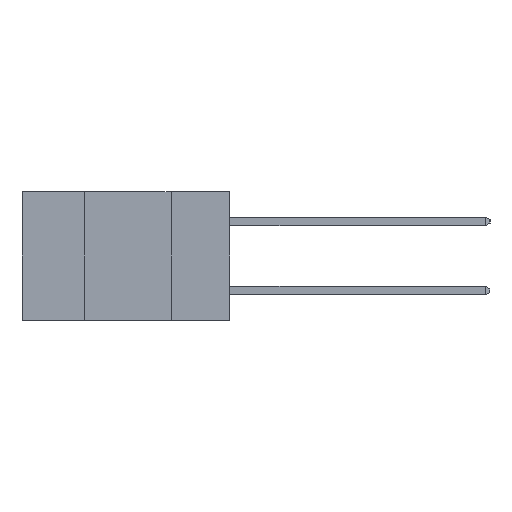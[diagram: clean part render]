
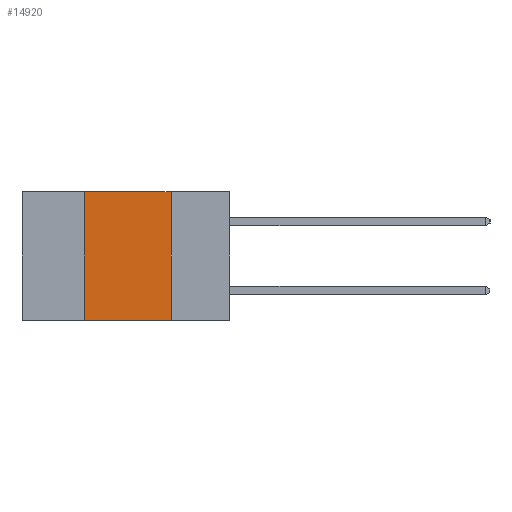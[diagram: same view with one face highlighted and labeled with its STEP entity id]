
A CAD part, left-side view. The second image highlights one B-rep face of the part: STEP entity #14920.
In plain terms, the highlighted planar face has unit normal (-1, 0, 0).
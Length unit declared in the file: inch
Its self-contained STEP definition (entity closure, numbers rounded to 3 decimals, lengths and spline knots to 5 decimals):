
#61 = DIRECTION ( 'NONE',  ( 0., 0., -1. ) ) ;
#88 = CARTESIAN_POINT ( 'NONE',  ( 0., 0.42, 0. ) ) ;
#108 = VERTEX_POINT ( 'NONE', #1842 ) ;
#618 = ORIENTED_EDGE ( 'NONE', *, *, #6790, .T. ) ;
#904 = EDGE_CURVE ( 'NONE', #108, #15260, #6940, .T. ) ;
#1454 = EDGE_CURVE ( 'NONE', #15260, #5382, #8753, .T. ) ;
#1842 = CARTESIAN_POINT ( 'NONE',  ( 0., 0.42, 0. ) ) ;
#1927 = CARTESIAN_POINT ( 'NONE',  ( 0., 0.42, -0.37 ) ) ;
#3386 = ORIENTED_EDGE ( 'NONE', *, *, #904, .F. ) ;
#3611 = CARTESIAN_POINT ( 'NONE',  ( 0., 0.17, -0.37 ) ) ;
#3631 = VERTEX_POINT ( 'NONE', #1927 ) ;
#4198 = PLANE ( 'NONE',  #15284 ) ;
#5382 = VERTEX_POINT ( 'NONE', #3611 ) ;
#5524 = CARTESIAN_POINT ( 'NONE',  ( 0., 0.6, 0. ) ) ;
#6143 = EDGE_LOOP ( 'NONE', ( #10988, #3386, #8619, #618 ) ) ;
#6790 = EDGE_CURVE ( 'NONE', #3631, #5382, #8629, .T. ) ;
#6885 = DIRECTION ( 'NONE',  ( 1., 0., 0. ) ) ;
#6940 = LINE ( 'NONE', #11953, #9926 ) ;
#7466 = CARTESIAN_POINT ( 'NONE',  ( 0., 0.17, 0. ) ) ;
#7942 = DIRECTION ( 'NONE',  ( 0., -1., 0. ) ) ;
#8619 = ORIENTED_EDGE ( 'NONE', *, *, #9367, .F. ) ;
#8629 = LINE ( 'NONE', #16247, #11973 ) ;
#8753 = LINE ( 'NONE', #16553, #11331 ) ;
#9367 = EDGE_CURVE ( 'NONE', #3631, #108, #9909, .T. ) ;
#9909 = LINE ( 'NONE', #88, #12899 ) ;
#9926 = VECTOR ( 'NONE', #7942, 39.37008 ) ;
#10988 = ORIENTED_EDGE ( 'NONE', *, *, #1454, .F. ) ;
#11331 = VECTOR ( 'NONE', #61, 39.37008 ) ;
#11953 = CARTESIAN_POINT ( 'NONE',  ( 0., 0.6, 0. ) ) ;
#11973 = VECTOR ( 'NONE', #14902, 39.37008 ) ;
#12882 = FACE_OUTER_BOUND ( 'NONE', #6143, .T. ) ;
#12899 = VECTOR ( 'NONE', #13016, 39.37008 ) ;
#13016 = DIRECTION ( 'NONE',  ( 0., 0., 1. ) ) ;
#14902 = DIRECTION ( 'NONE',  ( 0., -1., 0. ) ) ;
#14920 = ADVANCED_FACE ( 'NONE', ( #12882 ), #4198, .F. ) ;
#15260 = VERTEX_POINT ( 'NONE', #7466 ) ;
#15284 = AXIS2_PLACEMENT_3D ( 'NONE', #5524, #6885, #15946 ) ;
#15946 = DIRECTION ( 'NONE',  ( 0., 0., -1. ) ) ;
#16247 = CARTESIAN_POINT ( 'NONE',  ( 0., 0.6, -0.37 ) ) ;
#16553 = CARTESIAN_POINT ( 'NONE',  ( 0., 0.17, 0. ) ) ;
